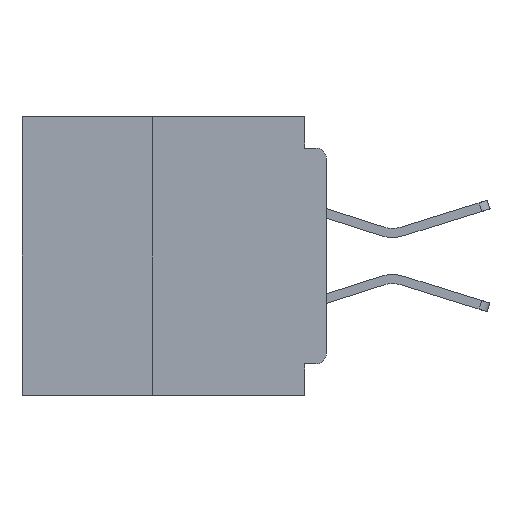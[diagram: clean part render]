
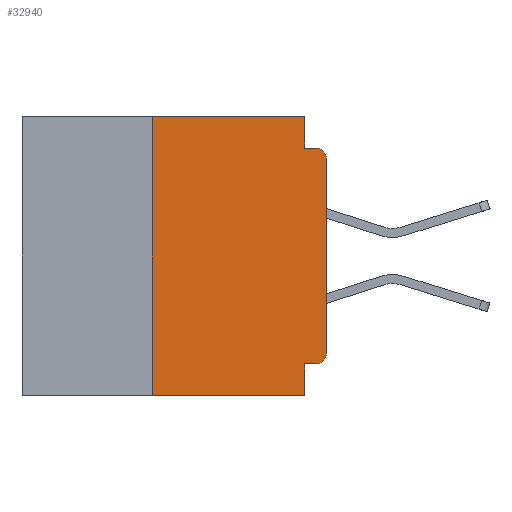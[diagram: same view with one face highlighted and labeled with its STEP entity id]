
A CAD part, left-side view. The second image highlights one B-rep face of the part: STEP entity #32940.
In plain terms, the highlighted planar face has unit normal (-1, 0, 0).
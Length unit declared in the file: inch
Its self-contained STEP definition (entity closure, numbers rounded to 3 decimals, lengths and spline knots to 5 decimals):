
#25 = EDGE_CURVE ( 'NONE', #10179, #13305, #29839, .T. ) ;
#353 = LINE ( 'NONE', #39058, #24162 ) ;
#1925 = VERTEX_POINT ( 'NONE', #20384 ) ;
#3584 = EDGE_CURVE ( 'NONE', #39287, #6114, #353, .T. ) ;
#4196 = LINE ( 'NONE', #42823, #26612 ) ;
#4672 = DIRECTION ( 'NONE',  ( 0., 0., -1. ) ) ;
#5879 = CARTESIAN_POINT ( 'NONE',  ( 0., 0.015, -0.34 ) ) ;
#6114 = VERTEX_POINT ( 'NONE', #24512 ) ;
#6433 = DIRECTION ( 'NONE',  ( -1., 0., 0. ) ) ;
#7104 = CIRCLE ( 'NONE', #36305, 0.015 ) ;
#8034 = VERTEX_POINT ( 'NONE', #24298 ) ;
#9189 = VERTEX_POINT ( 'NONE', #19957 ) ;
#9568 = EDGE_LOOP ( 'NONE', ( #41928, #31464, #22409, #23821, #13263, #16111, #17518, #55872, #46805, #16851 ) ) ;
#10179 = VERTEX_POINT ( 'NONE', #45203 ) ;
#10378 = DIRECTION ( 'NONE',  ( 0., 0., -1. ) ) ;
#11240 = VERTEX_POINT ( 'NONE', #38795 ) ;
#13263 = ORIENTED_EDGE ( 'NONE', *, *, #25, .F. ) ;
#13305 = VERTEX_POINT ( 'NONE', #22609 ) ;
#15443 = PLANE ( 'NONE',  #19397 ) ;
#15661 = VECTOR ( 'NONE', #27910, 39.37008 ) ;
#16111 = ORIENTED_EDGE ( 'NONE', *, *, #37867, .F. ) ;
#16851 = ORIENTED_EDGE ( 'NONE', *, *, #38206, .T. ) ;
#17329 = EDGE_CURVE ( 'NONE', #42913, #8034, #7104, .T. ) ;
#17518 = ORIENTED_EDGE ( 'NONE', *, *, #44322, .T. ) ;
#17954 = VECTOR ( 'NONE', #39083, 39.37008 ) ;
#18721 = CARTESIAN_POINT ( 'NONE',  ( 0., 0., 0. ) ) ;
#19037 = EDGE_CURVE ( 'NONE', #6114, #11240, #36793, .T. ) ;
#19397 = AXIS2_PLACEMENT_3D ( 'NONE', #42183, #46622, #19942 ) ;
#19824 = VECTOR ( 'NONE', #21580, 39.37008 ) ;
#19942 = DIRECTION ( 'NONE',  ( 0., 0., -1. ) ) ;
#19957 = CARTESIAN_POINT ( 'NONE',  ( 0., 0.031, -0.045 ) ) ;
#20228 = VERTEX_POINT ( 'NONE', #49019 ) ;
#20384 = CARTESIAN_POINT ( 'NONE',  ( 0., 0., -0.34 ) ) ;
#21580 = DIRECTION ( 'NONE',  ( 0., -1., 0. ) ) ;
#22409 = ORIENTED_EDGE ( 'NONE', *, *, #29123, .F. ) ;
#22609 = CARTESIAN_POINT ( 'NONE',  ( 0., 0.031, 0. ) ) ;
#23500 = EDGE_CURVE ( 'NONE', #13305, #9189, #32865, .T. ) ;
#23821 = ORIENTED_EDGE ( 'NONE', *, *, #23500, .F. ) ;
#24162 = VECTOR ( 'NONE', #39011, 39.37008 ) ;
#24298 = CARTESIAN_POINT ( 'NONE',  ( 0., 0.015, -0.045 ) ) ;
#24512 = CARTESIAN_POINT ( 'NONE',  ( 0., 0.031, -0.355 ) ) ;
#26612 = VECTOR ( 'NONE', #47262, 39.37008 ) ;
#27579 = LINE ( 'NONE', #18721, #15661 ) ;
#27910 = DIRECTION ( 'NONE',  ( 0., 0., 1. ) ) ;
#29123 = EDGE_CURVE ( 'NONE', #9189, #8034, #30307, .T. ) ;
#29302 = FACE_OUTER_BOUND ( 'NONE', #9568, .T. ) ;
#29839 = LINE ( 'NONE', #43316, #17954 ) ;
#30307 = LINE ( 'NONE', #48280, #19824 ) ;
#30820 = CARTESIAN_POINT ( 'NONE',  ( 0., 0.015, -0.355 ) ) ;
#31190 = CARTESIAN_POINT ( 'NONE',  ( 0., 0., -0.06 ) ) ;
#31462 = VECTOR ( 'NONE', #56457, 39.37008 ) ;
#31464 = ORIENTED_EDGE ( 'NONE', *, *, #17329, .T. ) ;
#32256 = CARTESIAN_POINT ( 'NONE',  ( 0., 0.437, -0.4 ) ) ;
#32865 = LINE ( 'NONE', #38551, #31462 ) ;
#32940 = ADVANCED_FACE ( 'NONE', ( #29302 ), #15443, .F. ) ;
#33198 = CARTESIAN_POINT ( 'NONE',  ( 0., 0.015, -0.06 ) ) ;
#34203 = AXIS2_PLACEMENT_3D ( 'NONE', #5879, #37145, #10378 ) ;
#35416 = VECTOR ( 'NONE', #4672, 39.37008 ) ;
#36305 = AXIS2_PLACEMENT_3D ( 'NONE', #33198, #6433, #37702 ) ;
#36793 = LINE ( 'NONE', #53852, #35416 ) ;
#37145 = DIRECTION ( 'NONE',  ( -1., 0., 0. ) ) ;
#37702 = DIRECTION ( 'NONE',  ( 0., 0., -1. ) ) ;
#37867 = EDGE_CURVE ( 'NONE', #20228, #10179, #4196, .T. ) ;
#38206 = EDGE_CURVE ( 'NONE', #39287, #1925, #55820, .T. ) ;
#38551 = CARTESIAN_POINT ( 'NONE',  ( 0., 0.031, 0. ) ) ;
#38795 = CARTESIAN_POINT ( 'NONE',  ( 0., 0.031, -0.4 ) ) ;
#39011 = DIRECTION ( 'NONE',  ( 0., 1., 0. ) ) ;
#39058 = CARTESIAN_POINT ( 'NONE',  ( 0., 0., -0.355 ) ) ;
#39083 = DIRECTION ( 'NONE',  ( 0., -1., 0. ) ) ;
#39287 = VERTEX_POINT ( 'NONE', #30820 ) ;
#40196 = LINE ( 'NONE', #32256, #49242 ) ;
#41928 = ORIENTED_EDGE ( 'NONE', *, *, #56248, .T. ) ;
#42183 = CARTESIAN_POINT ( 'NONE',  ( 0., 0.437, 0. ) ) ;
#42823 = CARTESIAN_POINT ( 'NONE',  ( 0., 0.25, -0.4 ) ) ;
#42913 = VERTEX_POINT ( 'NONE', #31190 ) ;
#43316 = CARTESIAN_POINT ( 'NONE',  ( 0., 0.437, 0. ) ) ;
#44322 = EDGE_CURVE ( 'NONE', #20228, #11240, #40196, .T. ) ;
#45203 = CARTESIAN_POINT ( 'NONE',  ( 0., 0.25, 0. ) ) ;
#45687 = DIRECTION ( 'NONE',  ( 0., -1., 0. ) ) ;
#46622 = DIRECTION ( 'NONE',  ( 1., 0., 0. ) ) ;
#46805 = ORIENTED_EDGE ( 'NONE', *, *, #3584, .F. ) ;
#47262 = DIRECTION ( 'NONE',  ( 0., 0., 1. ) ) ;
#48280 = CARTESIAN_POINT ( 'NONE',  ( 0., 0., -0.045 ) ) ;
#49019 = CARTESIAN_POINT ( 'NONE',  ( 0., 0.25, -0.4 ) ) ;
#49242 = VECTOR ( 'NONE', #45687, 39.37008 ) ;
#53852 = CARTESIAN_POINT ( 'NONE',  ( 0., 0.031, -0.4 ) ) ;
#55820 = CIRCLE ( 'NONE', #34203, 0.015 ) ;
#55872 = ORIENTED_EDGE ( 'NONE', *, *, #19037, .F. ) ;
#56248 = EDGE_CURVE ( 'NONE', #1925, #42913, #27579, .T. ) ;
#56457 = DIRECTION ( 'NONE',  ( 0., 0., -1. ) ) ;
